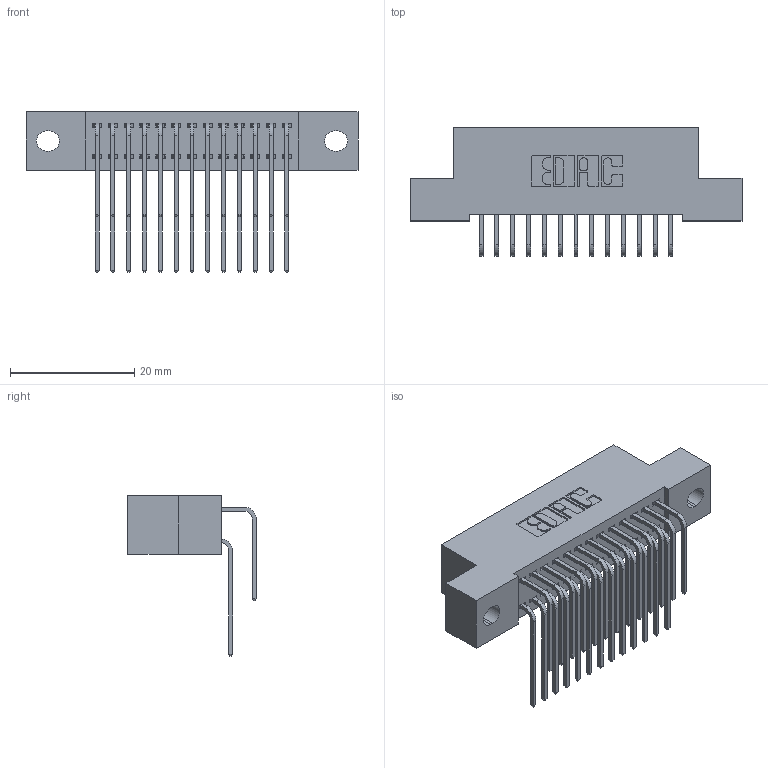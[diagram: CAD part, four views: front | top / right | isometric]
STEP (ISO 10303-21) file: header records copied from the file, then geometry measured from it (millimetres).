
FILE_DESCRIPTION (( 'STEP AP203' ), '1' );
FILE_NAME ('392-026-559-202.STEP', '2019-10-07T11:41:59', ( '' ), ( '' ), 'SwSTEP 2.0', 'SolidWorks 2016', '' );
FILE_SCHEMA (( 'CONFIG_CONTROL_DESIGN' ));
Length unit declared in the file: inch
Products named in the file (4): 342 Part_.128 Slot; 392-026-559-202; 345-292-001_558 559 Tail - 1; 345-292-001_559 Tail - 2
Assembly tree (27 placements, depth 2):
  392-026-559-202
    342 Part_.128 Slot
    345-292-001_558 559 Tail - 1  x13
    345-292-001_559 Tail - 2  x13
Bounding box: 53.34 x 20.64 x 25.78 mm (x, y, z)
Volume: 4753.2 mm3; surface area: 7460.4 mm2
Topology: 27 solids, 27 shells, 1518 faces, 4497 edges, 2962 vertices
Faces by surface type: plane 1058, cylinder 460
Entity records: 13901 total; most frequent: CARTESIAN_POINT 2389, ORIENTED_EDGE 2274, DIRECTION 2073, EDGE_CURVE 1137, VECTOR 969, LINE 969, VERTEX_POINT 754, AXIS2_PLACEMENT_3D 552
